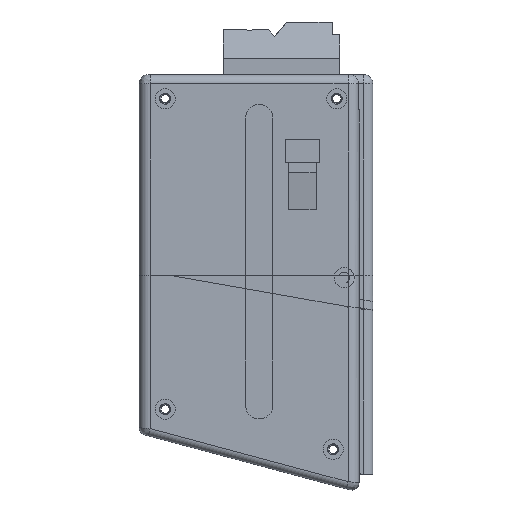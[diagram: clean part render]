
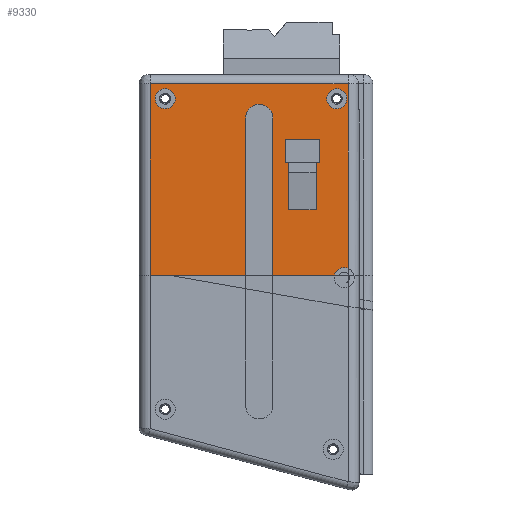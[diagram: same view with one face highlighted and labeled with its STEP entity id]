
A CAD part, front view. The second image highlights one B-rep face of the part: STEP entity #9330.
In plain terms, the highlighted planar face has unit normal (0, -1, 0).
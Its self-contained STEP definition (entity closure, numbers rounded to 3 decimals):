
#218=FACE_BOUND('',#1342,.T.);
#219=FACE_BOUND('',#1343,.T.);
#220=FACE_BOUND('',#1344,.T.);
#329=PLANE('',#9892);
#817=FACE_OUTER_BOUND('',#1341,.T.);
#1341=EDGE_LOOP('',(#8254,#8255,#8256,#8257,#8258,#8259,#8260,#8261,#8262));
#1342=EDGE_LOOP('',(#8263,#8264,#8265,#8266,#8267,#8268,#8269,#8270));
#1343=EDGE_LOOP('',(#8271));
#1344=EDGE_LOOP('',(#8272));
#1515=CIRCLE('',#9844,3.75);
#1528=CIRCLE('',#9885,2.75);
#1530=CIRCLE('',#9891,2.75);
#1531=CIRCLE('',#9893,2.75);
#2707=LINE('',#76826,#3269);
#2716=LINE('',#77154,#3278);
#2719=LINE('',#77165,#3281);
#2720=LINE('',#77168,#3282);
#2731=LINE('',#77207,#3293);
#2734=LINE('',#77212,#3296);
#2737=LINE('',#77217,#3299);
#2738=LINE('',#77220,#3300);
#2740=LINE('',#77223,#3302);
#2742=LINE('',#77227,#3304);
#2744=LINE('',#77231,#3306);
#2745=LINE('',#77233,#3307);
#2752=LINE('',#79215,#3314);
#2758=LINE('',#81118,#3320);
#2759=LINE('',#81119,#3321);
#3269=VECTOR('',#11235,10.);
#3278=VECTOR('',#11254,10.);
#3281=VECTOR('',#11263,10.);
#3282=VECTOR('',#11266,10.);
#3293=VECTOR('',#11291,10.);
#3296=VECTOR('',#11294,10.);
#3299=VECTOR('',#11299,10.);
#3300=VECTOR('',#11302,10.);
#3302=VECTOR('',#11306,10.);
#3304=VECTOR('',#11310,10.);
#3306=VECTOR('',#11314,10.);
#3307=VECTOR('',#11317,10.);
#3314=VECTOR('',#11354,10.);
#3320=VECTOR('',#11398,10.);
#3321=VECTOR('',#11399,10.);
#4181=VERTEX_POINT('',#76777);
#4185=VERTEX_POINT('',#76824);
#4207=VERTEX_POINT('',#77151);
#4208=VERTEX_POINT('',#77153);
#4209=VERTEX_POINT('',#77161);
#4210=VERTEX_POINT('',#77167);
#4220=VERTEX_POINT('',#77204);
#4221=VERTEX_POINT('',#77206);
#4222=VERTEX_POINT('',#77209);
#4223=VERTEX_POINT('',#77211);
#4224=VERTEX_POINT('',#77215);
#4225=VERTEX_POINT('',#77219);
#4226=VERTEX_POINT('',#77225);
#4227=VERTEX_POINT('',#77229);
#4235=VERTEX_POINT('',#79211);
#4239=VERTEX_POINT('',#80182);
#4241=VERTEX_POINT('',#81111);
#4242=VERTEX_POINT('',#81115);
#4243=VERTEX_POINT('',#81116);
#5501=EDGE_CURVE('',#4181,#4185,#2707,.T.);
#5534=EDGE_CURVE('',#4208,#4207,#2716,.T.);
#5537=EDGE_CURVE('',#4209,#4208,#1515,.T.);
#5539=EDGE_CURVE('',#4185,#4209,#2719,.T.);
#5540=EDGE_CURVE('',#4181,#4210,#2720,.T.);
#5555=EDGE_CURVE('',#4220,#4221,#2731,.T.);
#5558=EDGE_CURVE('',#4222,#4223,#2734,.T.);
#5561=EDGE_CURVE('',#4222,#4224,#2737,.T.);
#5562=EDGE_CURVE('',#4225,#4221,#2738,.T.);
#5564=EDGE_CURVE('',#4224,#4225,#2740,.T.);
#5566=EDGE_CURVE('',#4220,#4226,#2742,.T.);
#5568=EDGE_CURVE('',#4227,#4223,#2744,.T.);
#5569=EDGE_CURVE('',#4226,#4227,#2745,.T.);
#5594=EDGE_CURVE('',#4210,#4235,#2752,.T.);
#5604=EDGE_CURVE('',#4239,#4239,#1528,.T.);
#5610=EDGE_CURVE('',#4241,#4241,#1530,.T.);
#5612=EDGE_CURVE('',#4242,#4243,#1531,.T.);
#5613=EDGE_CURVE('',#4235,#4243,#2758,.T.);
#5614=EDGE_CURVE('',#4207,#4242,#2759,.T.);
#8254=ORIENTED_EDGE('',*,*,#5612,.T.);
#8255=ORIENTED_EDGE('',*,*,#5613,.F.);
#8256=ORIENTED_EDGE('',*,*,#5594,.F.);
#8257=ORIENTED_EDGE('',*,*,#5540,.F.);
#8258=ORIENTED_EDGE('',*,*,#5501,.T.);
#8259=ORIENTED_EDGE('',*,*,#5539,.T.);
#8260=ORIENTED_EDGE('',*,*,#5537,.T.);
#8261=ORIENTED_EDGE('',*,*,#5534,.T.);
#8262=ORIENTED_EDGE('',*,*,#5614,.T.);
#8263=ORIENTED_EDGE('',*,*,#5561,.T.);
#8264=ORIENTED_EDGE('',*,*,#5564,.T.);
#8265=ORIENTED_EDGE('',*,*,#5562,.T.);
#8266=ORIENTED_EDGE('',*,*,#5555,.F.);
#8267=ORIENTED_EDGE('',*,*,#5566,.T.);
#8268=ORIENTED_EDGE('',*,*,#5569,.T.);
#8269=ORIENTED_EDGE('',*,*,#5568,.T.);
#8270=ORIENTED_EDGE('',*,*,#5558,.F.);
#8271=ORIENTED_EDGE('',*,*,#5604,.T.);
#8272=ORIENTED_EDGE('',*,*,#5610,.T.);
#9330=ADVANCED_FACE('',(#817,#218,#219,#220),#329,.T.);
#9844=AXIS2_PLACEMENT_3D('',#77162,#11258,#11259);
#9885=AXIS2_PLACEMENT_3D('',#80183,#11378,#11379);
#9891=AXIS2_PLACEMENT_3D('',#81112,#11391,#11392);
#9892=AXIS2_PLACEMENT_3D('',#81114,#11394,#11395);
#9893=AXIS2_PLACEMENT_3D('',#81117,#11396,#11397);
#11235=DIRECTION('',(1.,0.,0.));
#11254=DIRECTION('',(0.,0.,-1.));
#11258=DIRECTION('center_axis',(0.,1.,0.));
#11259=DIRECTION('ref_axis',(1.,0.,0.));
#11263=DIRECTION('',(0.,0.,1.));
#11266=DIRECTION('',(0.,0.,1.));
#11291=DIRECTION('',(1.,0.,0.));
#11294=DIRECTION('',(1.,0.,0.));
#11299=DIRECTION('',(0.,0.,1.));
#11302=DIRECTION('',(0.,0.,-1.));
#11306=DIRECTION('',(1.,0.,0.));
#11310=DIRECTION('',(0.,0.,-1.));
#11314=DIRECTION('',(0.,0.,1.));
#11317=DIRECTION('',(-1.,0.,0.));
#11354=DIRECTION('',(1.,0.,0.));
#11378=DIRECTION('center_axis',(0.,1.,0.));
#11379=DIRECTION('ref_axis',(1.,0.,0.));
#11391=DIRECTION('center_axis',(0.,1.,0.));
#11392=DIRECTION('ref_axis',(1.,0.,0.));
#11394=DIRECTION('center_axis',(0.,-1.,0.));
#11395=DIRECTION('ref_axis',(1.,0.,0.));
#11396=DIRECTION('center_axis',(0.,1.,0.));
#11397=DIRECTION('ref_axis',(1.,0.,0.));
#11398=DIRECTION('',(0.,0.,-1.));
#11399=DIRECTION('',(1.,0.,0.));
#76777=CARTESIAN_POINT('',(339.124,-38.877,-21.513));
#76824=CARTESIAN_POINT('',(365.247,-38.877,-21.513));
#76826=CARTESIAN_POINT('',(362.285,-38.877,-21.513));
#77151=CARTESIAN_POINT('',(372.747,-38.877,-21.513));
#77153=CARTESIAN_POINT('',(372.747,-38.877,21.589));
#77154=CARTESIAN_POINT('',(372.747,-38.877,-19.67));
#77161=CARTESIAN_POINT('',(365.247,-38.877,21.589));
#77162=CARTESIAN_POINT('Origin',(368.997,-38.877,21.589));
#77165=CARTESIAN_POINT('',(365.247,-38.877,-59.));
#77167=CARTESIAN_POINT('',(339.124,-38.877,30.987));
#77168=CARTESIAN_POINT('',(339.124,-38.877,-60.891));
#77204=CARTESIAN_POINT('',(384.559,-38.877,9.391));
#77206=CARTESIAN_POINT('',(385.559,-38.877,9.391));
#77207=CARTESIAN_POINT('',(382.107,-38.877,9.391));
#77209=CARTESIAN_POINT('',(376.142,-38.877,9.391));
#77211=CARTESIAN_POINT('',(377.142,-38.877,9.391));
#77212=CARTESIAN_POINT('',(382.107,-38.877,9.391));
#77215=CARTESIAN_POINT('',(376.142,-38.877,15.814));
#77217=CARTESIAN_POINT('',(376.142,-38.877,-23.582));
#77219=CARTESIAN_POINT('',(385.559,-38.877,15.814));
#77220=CARTESIAN_POINT('',(385.559,-38.877,-23.582));
#77223=CARTESIAN_POINT('',(382.107,-38.877,15.814));
#77225=CARTESIAN_POINT('',(384.559,-38.877,-3.459));
#77227=CARTESIAN_POINT('',(384.559,-38.877,-32.194));
#77229=CARTESIAN_POINT('',(377.142,-38.877,-3.459));
#77231=CARTESIAN_POINT('',(377.142,-38.877,-27.194));
#77233=CARTESIAN_POINT('',(368.651,-38.877,-3.459));
#79211=CARTESIAN_POINT('',(393.335,-38.877,30.987));
#79215=CARTESIAN_POINT('',(372.807,-38.877,30.987));
#80182=CARTESIAN_POINT('',(340.493,-38.877,26.866));
#80183=CARTESIAN_POINT('Origin',(343.243,-38.877,26.866));
#81111=CARTESIAN_POINT('',(387.493,-38.877,26.866));
#81112=CARTESIAN_POINT('Origin',(390.243,-38.877,26.866));
#81114=CARTESIAN_POINT('Origin',(356.451,-38.877,-60.928));
#81115=CARTESIAN_POINT('',(389.564,-38.877,-21.513));
#81116=CARTESIAN_POINT('',(393.335,-38.877,-19.61));
#81117=CARTESIAN_POINT('Origin',(392.243,-38.877,-22.134));
#81118=CARTESIAN_POINT('',(393.335,-38.877,20.62));
#81119=CARTESIAN_POINT('',(362.285,-38.877,-21.513));
